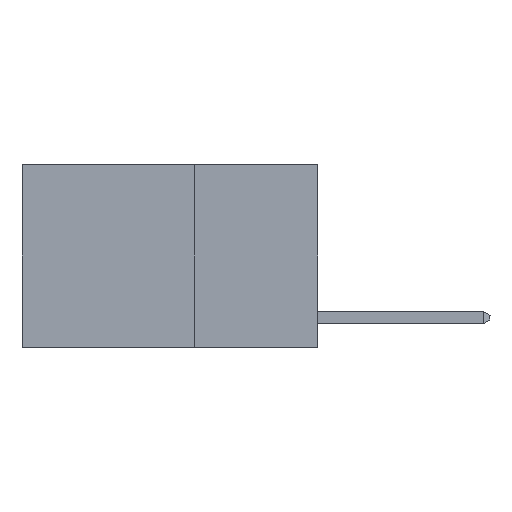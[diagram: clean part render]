
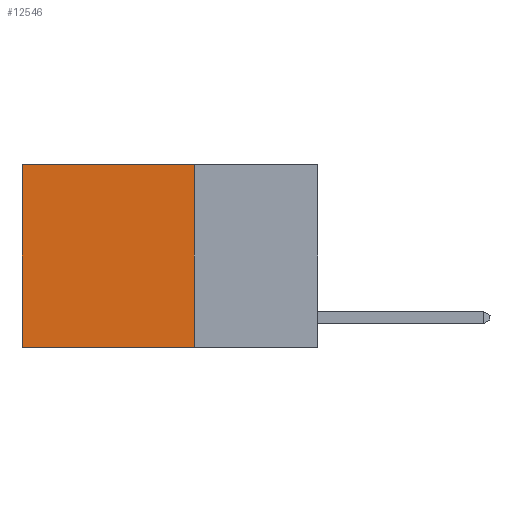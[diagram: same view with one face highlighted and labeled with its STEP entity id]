
A CAD part, left-side view. The second image highlights one B-rep face of the part: STEP entity #12546.
In plain terms, the highlighted planar face has unit normal (-1, 0, 0).
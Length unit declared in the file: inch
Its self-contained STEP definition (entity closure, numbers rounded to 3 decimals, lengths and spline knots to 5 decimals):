
#152 = VECTOR ( 'NONE', #14229, 39.37008 ) ;
#181 = EDGE_CURVE ( 'NONE', #11680, #13754, #8562, .T. ) ;
#255 = VECTOR ( 'NONE', #12813, 39.37008 ) ;
#314 = CARTESIAN_POINT ( 'NONE',  ( 0.2625, 0.25, -0.37 ) ) ;
#482 = DIRECTION ( 'NONE',  ( 0., 0., -1. ) ) ;
#1500 = CARTESIAN_POINT ( 'NONE',  ( 0.2625, 0.25, 0. ) ) ;
#1563 = LINE ( 'NONE', #13986, #6689 ) ;
#1575 = CARTESIAN_POINT ( 'NONE',  ( 0.2625, 0.25, 0. ) ) ;
#1822 = EDGE_LOOP ( 'NONE', ( #7817, #9227, #4212, #8236 ) ) ;
#3044 = VERTEX_POINT ( 'NONE', #3774 ) ;
#3446 = EDGE_CURVE ( 'NONE', #10309, #13754, #8024, .T. ) ;
#3519 = CARTESIAN_POINT ( 'NONE',  ( 0.2625, 0.6, 0. ) ) ;
#3535 = FACE_OUTER_BOUND ( 'NONE', #1822, .T. ) ;
#3774 = CARTESIAN_POINT ( 'NONE',  ( 0.2625, 0.25, 0. ) ) ;
#4212 = ORIENTED_EDGE ( 'NONE', *, *, #5437, .F. ) ;
#5139 = LINE ( 'NONE', #1575, #9905 ) ;
#5437 = EDGE_CURVE ( 'NONE', #3044, #10309, #5139, .T. ) ;
#6452 = CARTESIAN_POINT ( 'NONE',  ( 0.2625, 0.6, 0. ) ) ;
#6689 = VECTOR ( 'NONE', #13912, 39.37008 ) ;
#7026 = EDGE_CURVE ( 'NONE', #3044, #11680, #1563, .T. ) ;
#7817 = ORIENTED_EDGE ( 'NONE', *, *, #181, .T. ) ;
#8024 = LINE ( 'NONE', #314, #255 ) ;
#8236 = ORIENTED_EDGE ( 'NONE', *, *, #7026, .T. ) ;
#8562 = LINE ( 'NONE', #6452, #152 ) ;
#9063 = DIRECTION ( 'NONE',  ( 0., 0., -1. ) ) ;
#9227 = ORIENTED_EDGE ( 'NONE', *, *, #3446, .F. ) ;
#9905 = VECTOR ( 'NONE', #482, 39.37008 ) ;
#10294 = PLANE ( 'NONE',  #11649 ) ;
#10309 = VERTEX_POINT ( 'NONE', #14064 ) ;
#10806 = CARTESIAN_POINT ( 'NONE',  ( 0.2625, 0.6, -0.37 ) ) ;
#11370 = DIRECTION ( 'NONE',  ( 1., 0., 0. ) ) ;
#11649 = AXIS2_PLACEMENT_3D ( 'NONE', #1500, #11370, #9063 ) ;
#11680 = VERTEX_POINT ( 'NONE', #3519 ) ;
#12546 = ADVANCED_FACE ( 'NONE', ( #3535 ), #10294, .F. ) ;
#12813 = DIRECTION ( 'NONE',  ( 0., 1., 0. ) ) ;
#13754 = VERTEX_POINT ( 'NONE', #10806 ) ;
#13912 = DIRECTION ( 'NONE',  ( 0., 1., 0. ) ) ;
#13986 = CARTESIAN_POINT ( 'NONE',  ( 0.2625, 0.25, 0. ) ) ;
#14064 = CARTESIAN_POINT ( 'NONE',  ( 0.2625, 0.25, -0.37 ) ) ;
#14229 = DIRECTION ( 'NONE',  ( 0., 0., -1. ) ) ;
